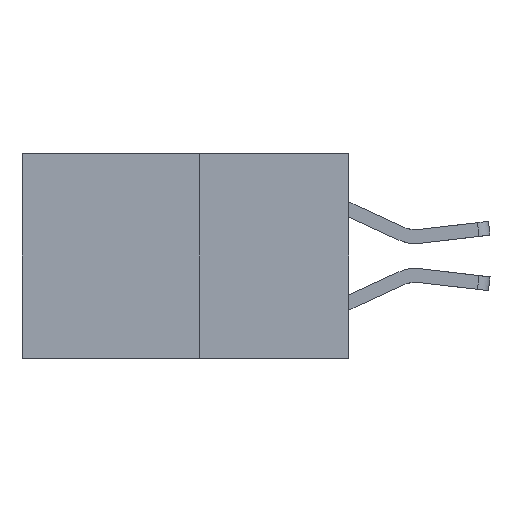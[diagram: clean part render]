
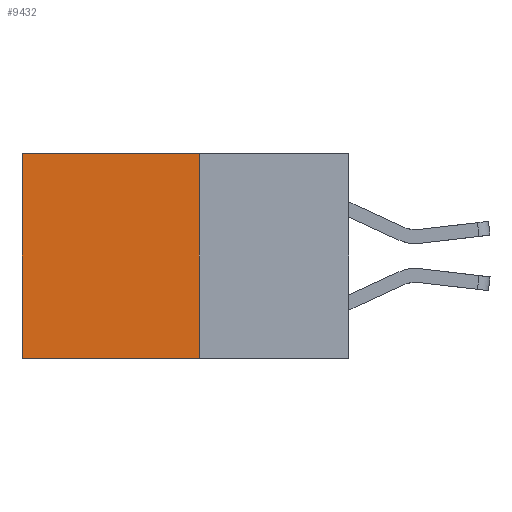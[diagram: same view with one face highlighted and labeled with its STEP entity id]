
A CAD part, left-side view. The second image highlights one B-rep face of the part: STEP entity #9432.
In plain terms, the highlighted planar face has unit normal (-1, 0, 0).
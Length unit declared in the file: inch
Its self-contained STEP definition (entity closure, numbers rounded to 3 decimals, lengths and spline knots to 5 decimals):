
#68 = EDGE_CURVE ( 'NONE', #709, #6920, #1071, .T. ) ;
#305 = VECTOR ( 'NONE', #1273, 39.37008 ) ;
#381 = LINE ( 'NONE', #5995, #4402 ) ;
#420 = VERTEX_POINT ( 'NONE', #6731 ) ;
#599 = EDGE_CURVE ( 'NONE', #420, #10223, #5083, .T. ) ;
#709 = VERTEX_POINT ( 'NONE', #3579 ) ;
#759 = EDGE_LOOP ( 'NONE', ( #9164, #6198, #9888, #2583 ) ) ;
#1071 = LINE ( 'NONE', #3819, #5352 ) ;
#1101 = CARTESIAN_POINT ( 'NONE',  ( 0.277, 0.59, -0.37 ) ) ;
#1273 = DIRECTION ( 'NONE',  ( 0., 0., -1. ) ) ;
#2583 = ORIENTED_EDGE ( 'NONE', *, *, #6884, .T. ) ;
#2593 = VECTOR ( 'NONE', #5969, 39.37008 ) ;
#2895 = DIRECTION ( 'NONE',  ( 1., 0., 0. ) ) ;
#3528 = CARTESIAN_POINT ( 'NONE',  ( 0.277, 0.27, 0. ) ) ;
#3579 = CARTESIAN_POINT ( 'NONE',  ( 0.277, 0.27, 0. ) ) ;
#3801 = DIRECTION ( 'NONE',  ( 0., 0., -1. ) ) ;
#3819 = CARTESIAN_POINT ( 'NONE',  ( 0.277, 0.27, -0.37 ) ) ;
#4166 = AXIS2_PLACEMENT_3D ( 'NONE', #8486, #2895, #8518 ) ;
#4402 = VECTOR ( 'NONE', #5181, 39.37008 ) ;
#4746 = CARTESIAN_POINT ( 'NONE',  ( 0.277, 0.59, -0.37 ) ) ;
#5083 = LINE ( 'NONE', #1101, #305 ) ;
#5181 = DIRECTION ( 'NONE',  ( 0., 1., 0. ) ) ;
#5352 = VECTOR ( 'NONE', #3801, 39.37008 ) ;
#5969 = DIRECTION ( 'NONE',  ( 0., 1., 0. ) ) ;
#5995 = CARTESIAN_POINT ( 'NONE',  ( 0.277, 0.27, -0.37 ) ) ;
#6101 = PLANE ( 'NONE',  #4166 ) ;
#6198 = ORIENTED_EDGE ( 'NONE', *, *, #9909, .F. ) ;
#6731 = CARTESIAN_POINT ( 'NONE',  ( 0.277, 0.59, 0. ) ) ;
#6803 = FACE_OUTER_BOUND ( 'NONE', #759, .T. ) ;
#6877 = LINE ( 'NONE', #3528, #2593 ) ;
#6884 = EDGE_CURVE ( 'NONE', #709, #420, #6877, .T. ) ;
#6920 = VERTEX_POINT ( 'NONE', #9228 ) ;
#8486 = CARTESIAN_POINT ( 'NONE',  ( 0.277, 0.27, -0.37 ) ) ;
#8518 = DIRECTION ( 'NONE',  ( 0., 0., -1. ) ) ;
#9164 = ORIENTED_EDGE ( 'NONE', *, *, #599, .T. ) ;
#9228 = CARTESIAN_POINT ( 'NONE',  ( 0.277, 0.27, -0.37 ) ) ;
#9432 = ADVANCED_FACE ( 'NONE', ( #6803 ), #6101, .F. ) ;
#9888 = ORIENTED_EDGE ( 'NONE', *, *, #68, .F. ) ;
#9909 = EDGE_CURVE ( 'NONE', #6920, #10223, #381, .T. ) ;
#10223 = VERTEX_POINT ( 'NONE', #4746 ) ;
